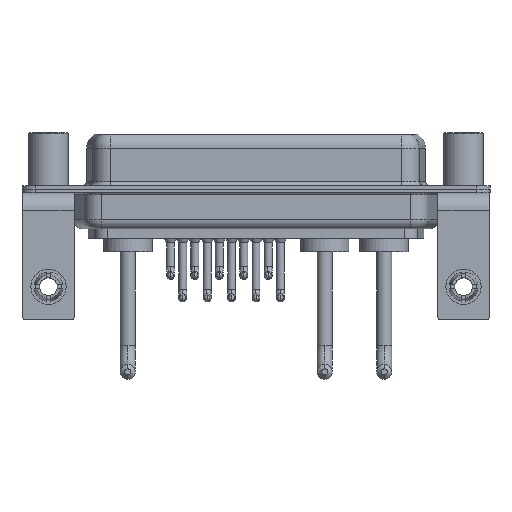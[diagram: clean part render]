
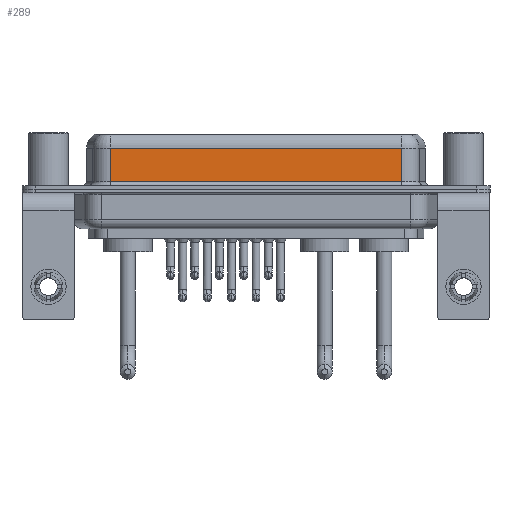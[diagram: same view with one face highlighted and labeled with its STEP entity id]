
A CAD part, front view. The second image highlights one B-rep face of the part: STEP entity #289.
In plain terms, the highlighted planar face has unit normal (0, -1, 0).
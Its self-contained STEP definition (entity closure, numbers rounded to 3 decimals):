
#289 = ADVANCED_FACE ( 'NONE', ( #13338 ), #8041, .F. ) ;
#678 = VERTEX_POINT ( 'NONE', #3814 ) ;
#1140 = VECTOR ( 'NONE', #21885, 1000. ) ;
#1606 = CARTESIAN_POINT ( 'NONE',  ( 7.013, -3.95, 4.65 ) ) ;
#1976 = CARTESIAN_POINT ( 'NONE',  ( 40.037, -3.95, 4.65 ) ) ;
#2734 = CARTESIAN_POINT ( 'NONE',  ( 7.013, -3.95, 0.9 ) ) ;
#2844 = LINE ( 'NONE', #8110, #15955 ) ;
#3814 = CARTESIAN_POINT ( 'NONE',  ( 40.037, -3.95, 4.65 ) ) ;
#4061 = DIRECTION ( 'NONE',  ( 0., 1., 0. ) ) ;
#5038 = DIRECTION ( 'NONE',  ( -1., 0., 0. ) ) ;
#6054 = EDGE_CURVE ( 'NONE', #678, #17565, #10866, .T. ) ;
#6259 = VECTOR ( 'NONE', #5038, 1000. ) ;
#7142 = LINE ( 'NONE', #14714, #1140 ) ;
#8041 = PLANE ( 'NONE',  #9286 ) ;
#8110 = CARTESIAN_POINT ( 'NONE',  ( 40.037, -3.95, 0.9 ) ) ;
#8193 = DIRECTION ( 'NONE',  ( 0., 0., -1. ) ) ;
#8424 = CARTESIAN_POINT ( 'NONE',  ( 40.037, -3.95, 6.4 ) ) ;
#8751 = EDGE_CURVE ( 'NONE', #678, #12866, #17487, .T. ) ;
#9286 = AXIS2_PLACEMENT_3D ( 'NONE', #15228, #4061, #9454 ) ;
#9454 = DIRECTION ( 'NONE',  ( 0., 0., 1. ) ) ;
#10266 = CARTESIAN_POINT ( 'NONE',  ( 40.037, -3.95, 0.9 ) ) ;
#10866 = LINE ( 'NONE', #1976, #6259 ) ;
#11151 = EDGE_CURVE ( 'NONE', #17565, #11356, #7142, .T. ) ;
#11356 = VERTEX_POINT ( 'NONE', #2734 ) ;
#11369 = ORIENTED_EDGE ( 'NONE', *, *, #19537, .T. ) ;
#11701 = EDGE_LOOP ( 'NONE', ( #22513, #21647, #14803, #11369 ) ) ;
#12866 = VERTEX_POINT ( 'NONE', #10266 ) ;
#13338 = FACE_OUTER_BOUND ( 'NONE', #11701, .T. ) ;
#13382 = VECTOR ( 'NONE', #8193, 1000. ) ;
#14714 = CARTESIAN_POINT ( 'NONE',  ( 7.013, -3.95, 6.4 ) ) ;
#14803 = ORIENTED_EDGE ( 'NONE', *, *, #11151, .T. ) ;
#15228 = CARTESIAN_POINT ( 'NONE',  ( 40.037, -3.95, 6.4 ) ) ;
#15955 = VECTOR ( 'NONE', #18702, 1000. ) ;
#17487 = LINE ( 'NONE', #8424, #13382 ) ;
#17565 = VERTEX_POINT ( 'NONE', #1606 ) ;
#18702 = DIRECTION ( 'NONE',  ( 1., 0., 0. ) ) ;
#19537 = EDGE_CURVE ( 'NONE', #11356, #12866, #2844, .T. ) ;
#21647 = ORIENTED_EDGE ( 'NONE', *, *, #6054, .T. ) ;
#21885 = DIRECTION ( 'NONE',  ( 0., 0., -1. ) ) ;
#22513 = ORIENTED_EDGE ( 'NONE', *, *, #8751, .F. ) ;
